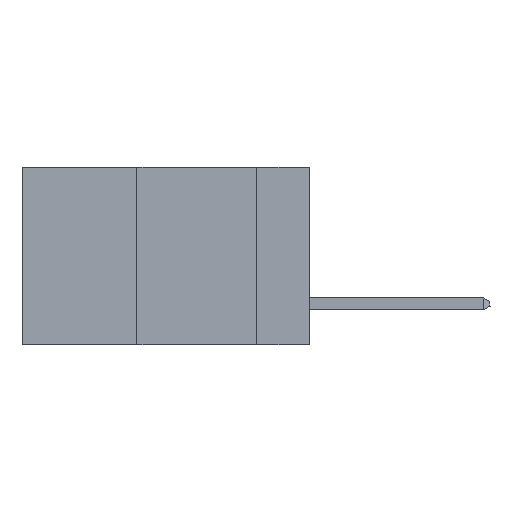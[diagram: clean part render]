
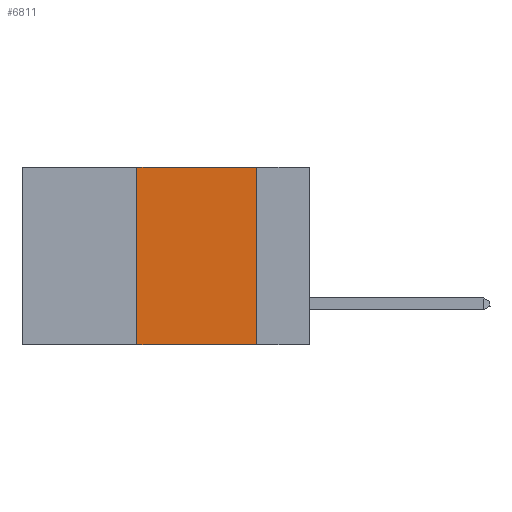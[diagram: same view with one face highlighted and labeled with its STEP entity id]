
A CAD part, left-side view. The second image highlights one B-rep face of the part: STEP entity #6811.
In plain terms, the highlighted planar face has unit normal (-1, 0, 0).
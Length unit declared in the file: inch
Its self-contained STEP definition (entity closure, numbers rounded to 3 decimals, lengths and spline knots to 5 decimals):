
#706 = CARTESIAN_POINT ( 'NONE',  ( 0., 0.11, 0. ) ) ;
#844 = LINE ( 'NONE', #706, #22578 ) ;
#2294 = EDGE_CURVE ( 'NONE', #11928, #15016, #19885, .T. ) ;
#3339 = VECTOR ( 'NONE', #11079, 39.37008 ) ;
#3884 = LINE ( 'NONE', #14742, #3339 ) ;
#4465 = VERTEX_POINT ( 'NONE', #16387 ) ;
#5471 = FACE_OUTER_BOUND ( 'NONE', #9123, .T. ) ;
#6298 = DIRECTION ( 'NONE',  ( 0., 0., -1. ) ) ;
#6811 = ADVANCED_FACE ( 'NONE', ( #5471 ), #8994, .F. ) ;
#7323 = CARTESIAN_POINT ( 'NONE',  ( 0., 0.6, 0. ) ) ;
#8300 = DIRECTION ( 'NONE',  ( 0., 0., 1. ) ) ;
#8633 = VECTOR ( 'NONE', #8300, 39.37008 ) ;
#8994 = PLANE ( 'NONE',  #17681 ) ;
#9123 = EDGE_LOOP ( 'NONE', ( #16680, #22149, #17680, #10042 ) ) ;
#10042 = ORIENTED_EDGE ( 'NONE', *, *, #2294, .T. ) ;
#10714 = VERTEX_POINT ( 'NONE', #16226 ) ;
#11079 = DIRECTION ( 'NONE',  ( 0., -1., 0. ) ) ;
#11554 = CARTESIAN_POINT ( 'NONE',  ( 0., 0.6, -0.37 ) ) ;
#11721 = DIRECTION ( 'NONE',  ( 0., -1., 0. ) ) ;
#11928 = VERTEX_POINT ( 'NONE', #13701 ) ;
#13509 = LINE ( 'NONE', #15439, #8633 ) ;
#13701 = CARTESIAN_POINT ( 'NONE',  ( 0., 0.36, -0.37 ) ) ;
#14136 = VECTOR ( 'NONE', #11721, 39.37008 ) ;
#14654 = DIRECTION ( 'NONE',  ( 0., 0., -1. ) ) ;
#14742 = CARTESIAN_POINT ( 'NONE',  ( 0., 0.6, 0. ) ) ;
#15016 = VERTEX_POINT ( 'NONE', #18133 ) ;
#15439 = CARTESIAN_POINT ( 'NONE',  ( 0., 0.36, 0. ) ) ;
#16226 = CARTESIAN_POINT ( 'NONE',  ( 0., 0.36, 0. ) ) ;
#16387 = CARTESIAN_POINT ( 'NONE',  ( 0., 0.11, 0. ) ) ;
#16680 = ORIENTED_EDGE ( 'NONE', *, *, #18398, .F. ) ;
#16759 = EDGE_CURVE ( 'NONE', #11928, #10714, #13509, .T. ) ;
#17680 = ORIENTED_EDGE ( 'NONE', *, *, #16759, .F. ) ;
#17681 = AXIS2_PLACEMENT_3D ( 'NONE', #7323, #23390, #14654 ) ;
#18133 = CARTESIAN_POINT ( 'NONE',  ( 0., 0.11, -0.37 ) ) ;
#18398 = EDGE_CURVE ( 'NONE', #4465, #15016, #844, .T. ) ;
#19885 = LINE ( 'NONE', #11554, #14136 ) ;
#20223 = EDGE_CURVE ( 'NONE', #10714, #4465, #3884, .T. ) ;
#22149 = ORIENTED_EDGE ( 'NONE', *, *, #20223, .F. ) ;
#22578 = VECTOR ( 'NONE', #6298, 39.37008 ) ;
#23390 = DIRECTION ( 'NONE',  ( 1., 0., 0. ) ) ;
